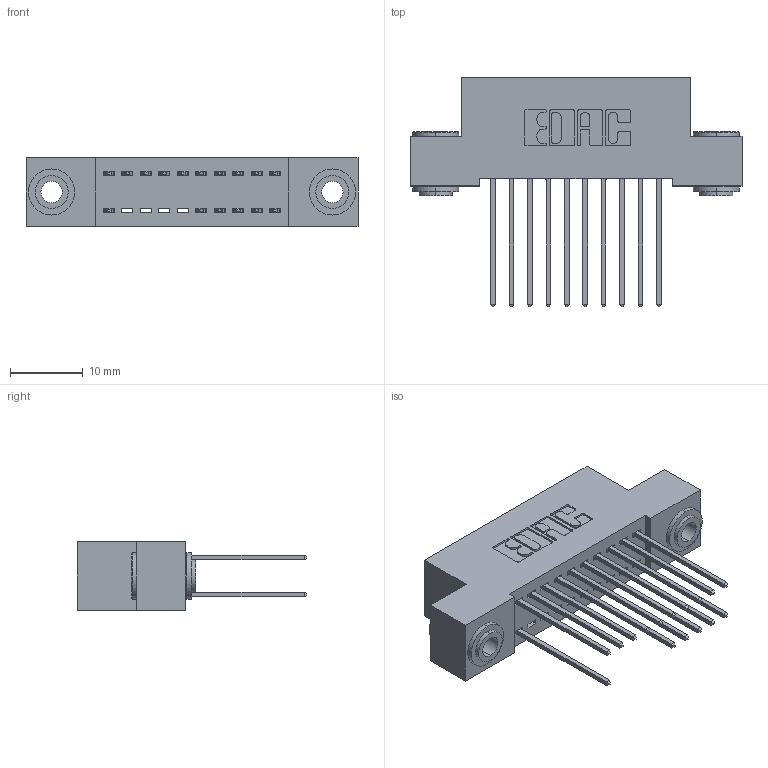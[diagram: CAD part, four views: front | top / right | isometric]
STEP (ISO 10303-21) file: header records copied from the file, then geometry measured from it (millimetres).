
FILE_DESCRIPTION (( 'STEP AP203' ), '1' );
FILE_NAME ('392-020-542-203.STEP', '2018-08-15T06:48:25', ( '' ), ( '' ), 'SwSTEP 2.0', 'SolidWorks 2016', '' );
FILE_SCHEMA (( 'CONFIG_CONTROL_DESIGN' ));
Length unit declared in the file: inch
Products named in the file (4): 342-250-002_345-250-002-102; 392-020-542-203; 342 Part_.156 TH; 345-292-001_345-293-142
Assembly tree (19 placements, depth 2):
  392-020-542-203
    342 Part_.156 TH
    345-292-001_345-293-142  x16
    342-250-002_345-250-002-102  x2
Bounding box: 45.72 x 31.63 x 9.4 mm (x, y, z)
Volume: 4017.9 mm3; surface area: 6101.5 mm2
Topology: 19 solids, 19 shells, 1004 faces, 2939 edges, 1934 vertices
Faces by surface type: plane 676, cylinder 320, cone 8
Entity records: 10980 total; most frequent: CARTESIAN_POINT 1849, ORIENTED_EDGE 1782, DIRECTION 1665, EDGE_CURVE 891, VECTOR 739, LINE 739, VERTEX_POINT 590, AXIS2_PLACEMENT_3D 463
